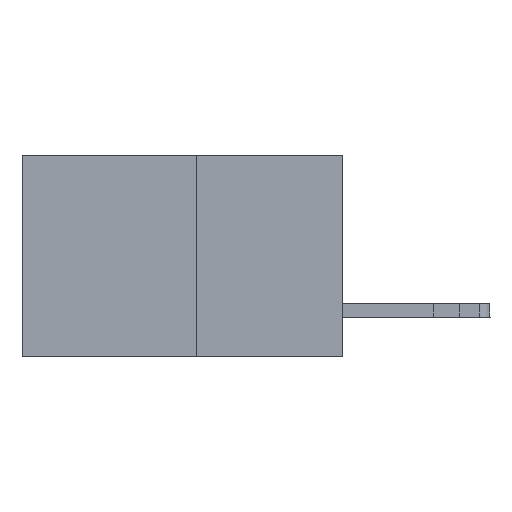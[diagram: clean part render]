
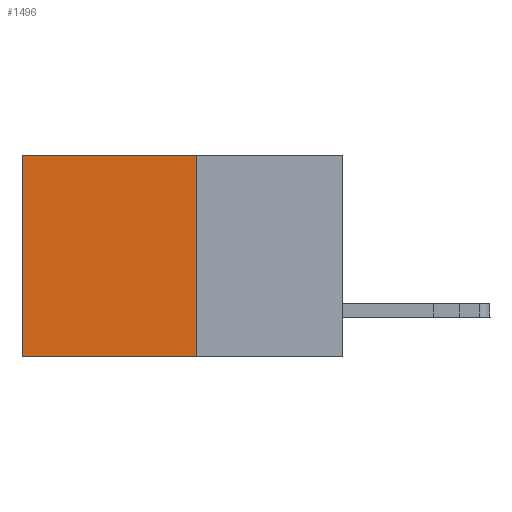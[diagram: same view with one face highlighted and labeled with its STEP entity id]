
A CAD part, left-side view. The second image highlights one B-rep face of the part: STEP entity #1496.
In plain terms, the highlighted planar face has unit normal (-1, 0, 0).
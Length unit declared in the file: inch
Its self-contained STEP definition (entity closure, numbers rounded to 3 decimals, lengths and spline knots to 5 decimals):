
#368 = ORIENTED_EDGE ( 'NONE', *, *, #9325, .F. ) ;
#745 = VECTOR ( 'NONE', #21692, 39.37008 ) ;
#1496 = ADVANCED_FACE ( 'NONE', ( #16242 ), #2337, .F. ) ;
#2337 = PLANE ( 'NONE',  #14533 ) ;
#2495 = CARTESIAN_POINT ( 'NONE',  ( 0.277, 0.59, -0.37 ) ) ;
#3734 = VECTOR ( 'NONE', #22225, 39.37008 ) ;
#4391 = LINE ( 'NONE', #8224, #3734 ) ;
#4705 = VECTOR ( 'NONE', #18908, 39.37008 ) ;
#4806 = CARTESIAN_POINT ( 'NONE',  ( 0.277, 0.27, -0.37 ) ) ;
#5416 = CARTESIAN_POINT ( 'NONE',  ( 0.277, 0.59, -0.37 ) ) ;
#5541 = LINE ( 'NONE', #19677, #745 ) ;
#5790 = ORIENTED_EDGE ( 'NONE', *, *, #22822, .T. ) ;
#6088 = DIRECTION ( 'NONE',  ( 0., 0., -1. ) ) ;
#7454 = DIRECTION ( 'NONE',  ( 0., 0., -1. ) ) ;
#8224 = CARTESIAN_POINT ( 'NONE',  ( 0.277, 0.27, -0.37 ) ) ;
#8453 = VERTEX_POINT ( 'NONE', #22847 ) ;
#8593 = LINE ( 'NONE', #5416, #9227 ) ;
#9227 = VECTOR ( 'NONE', #7454, 39.37008 ) ;
#9325 = EDGE_CURVE ( 'NONE', #12418, #13048, #4391, .T. ) ;
#9496 = EDGE_CURVE ( 'NONE', #13048, #18074, #14796, .T. ) ;
#9568 = ORIENTED_EDGE ( 'NONE', *, *, #24331, .T. ) ;
#12418 = VERTEX_POINT ( 'NONE', #25004 ) ;
#12763 = EDGE_LOOP ( 'NONE', ( #9568, #18696, #368, #5790 ) ) ;
#13048 = VERTEX_POINT ( 'NONE', #25249 ) ;
#14533 = AXIS2_PLACEMENT_3D ( 'NONE', #20045, #24934, #6088 ) ;
#14796 = LINE ( 'NONE', #4806, #4705 ) ;
#16242 = FACE_OUTER_BOUND ( 'NONE', #12763, .T. ) ;
#18074 = VERTEX_POINT ( 'NONE', #2495 ) ;
#18696 = ORIENTED_EDGE ( 'NONE', *, *, #9496, .F. ) ;
#18908 = DIRECTION ( 'NONE',  ( 0., 1., 0. ) ) ;
#19677 = CARTESIAN_POINT ( 'NONE',  ( 0.277, 0.27, 0. ) ) ;
#20045 = CARTESIAN_POINT ( 'NONE',  ( 0.277, 0.27, -0.37 ) ) ;
#21692 = DIRECTION ( 'NONE',  ( 0., 1., 0. ) ) ;
#22225 = DIRECTION ( 'NONE',  ( 0., 0., -1. ) ) ;
#22822 = EDGE_CURVE ( 'NONE', #12418, #8453, #5541, .T. ) ;
#22847 = CARTESIAN_POINT ( 'NONE',  ( 0.277, 0.59, 0. ) ) ;
#24331 = EDGE_CURVE ( 'NONE', #8453, #18074, #8593, .T. ) ;
#24934 = DIRECTION ( 'NONE',  ( 1., 0., 0. ) ) ;
#25004 = CARTESIAN_POINT ( 'NONE',  ( 0.277, 0.27, 0. ) ) ;
#25249 = CARTESIAN_POINT ( 'NONE',  ( 0.277, 0.27, -0.37 ) ) ;
